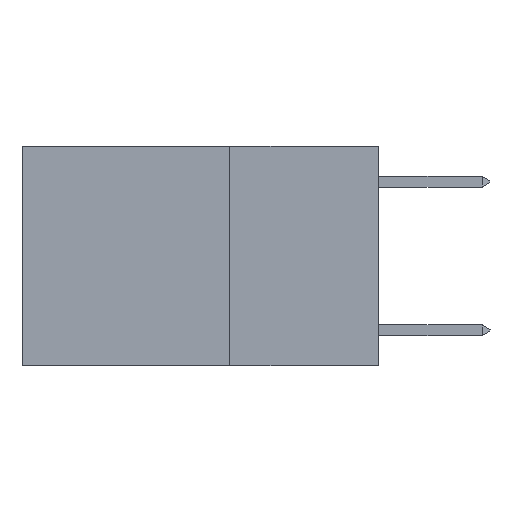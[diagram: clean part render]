
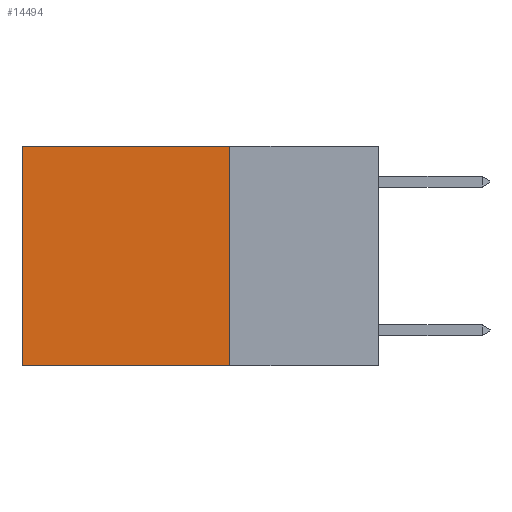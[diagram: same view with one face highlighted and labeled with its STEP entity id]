
A CAD part, left-side view. The second image highlights one B-rep face of the part: STEP entity #14494.
In plain terms, the highlighted planar face has unit normal (-1, 0, 0).
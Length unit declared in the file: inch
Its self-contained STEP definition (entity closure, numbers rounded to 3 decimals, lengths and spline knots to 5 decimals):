
#116 = AXIS2_PLACEMENT_3D ( 'NONE', #11566, #9330, #2612 ) ;
#146 = CARTESIAN_POINT ( 'NONE',  ( 0.2625, 0.25, 0. ) ) ;
#236 = PLANE ( 'NONE',  #116 ) ;
#1481 = LINE ( 'NONE', #8869, #2019 ) ;
#1498 = VERTEX_POINT ( 'NONE', #1998 ) ;
#1517 = ORIENTED_EDGE ( 'NONE', *, *, #3889, .T. ) ;
#1998 = CARTESIAN_POINT ( 'NONE',  ( 0.2625, 0.6, 0. ) ) ;
#2019 = VECTOR ( 'NONE', #7646, 39.37008 ) ;
#2323 = EDGE_CURVE ( 'NONE', #1498, #12649, #13516, .T. ) ;
#2612 = DIRECTION ( 'NONE',  ( 0., 0., -1. ) ) ;
#2726 = CARTESIAN_POINT ( 'NONE',  ( 0.2625, 0.6, 0. ) ) ;
#3119 = EDGE_CURVE ( 'NONE', #4940, #3930, #12803, .T. ) ;
#3484 = EDGE_LOOP ( 'NONE', ( #6771, #5141, #11082, #1517 ) ) ;
#3889 = EDGE_CURVE ( 'NONE', #4940, #1498, #1481, .T. ) ;
#3930 = VERTEX_POINT ( 'NONE', #10195 ) ;
#4091 = DIRECTION ( 'NONE',  ( 0., 1., 0. ) ) ;
#4475 = LINE ( 'NONE', #12823, #7286 ) ;
#4940 = VERTEX_POINT ( 'NONE', #8406 ) ;
#5141 = ORIENTED_EDGE ( 'NONE', *, *, #5424, .F. ) ;
#5424 = EDGE_CURVE ( 'NONE', #3930, #12649, #4475, .T. ) ;
#6205 = DIRECTION ( 'NONE',  ( 0., 0., -1. ) ) ;
#6771 = ORIENTED_EDGE ( 'NONE', *, *, #2323, .T. ) ;
#7286 = VECTOR ( 'NONE', #4091, 39.37008 ) ;
#7646 = DIRECTION ( 'NONE',  ( 0., 1., 0. ) ) ;
#8046 = FACE_OUTER_BOUND ( 'NONE', #3484, .T. ) ;
#8406 = CARTESIAN_POINT ( 'NONE',  ( 0.2625, 0.25, 0. ) ) ;
#8869 = CARTESIAN_POINT ( 'NONE',  ( 0.2625, 0.25, 0. ) ) ;
#9263 = VECTOR ( 'NONE', #10584, 39.37008 ) ;
#9330 = DIRECTION ( 'NONE',  ( 1., 0., 0. ) ) ;
#10195 = CARTESIAN_POINT ( 'NONE',  ( 0.2625, 0.25, -0.37 ) ) ;
#10584 = DIRECTION ( 'NONE',  ( 0., 0., -1. ) ) ;
#10841 = VECTOR ( 'NONE', #6205, 39.37008 ) ;
#11082 = ORIENTED_EDGE ( 'NONE', *, *, #3119, .F. ) ;
#11537 = CARTESIAN_POINT ( 'NONE',  ( 0.2625, 0.6, -0.37 ) ) ;
#11566 = CARTESIAN_POINT ( 'NONE',  ( 0.2625, 0.25, 0. ) ) ;
#12649 = VERTEX_POINT ( 'NONE', #11537 ) ;
#12803 = LINE ( 'NONE', #146, #10841 ) ;
#12823 = CARTESIAN_POINT ( 'NONE',  ( 0.2625, 0.25, -0.37 ) ) ;
#13516 = LINE ( 'NONE', #2726, #9263 ) ;
#14494 = ADVANCED_FACE ( 'NONE', ( #8046 ), #236, .F. ) ;
